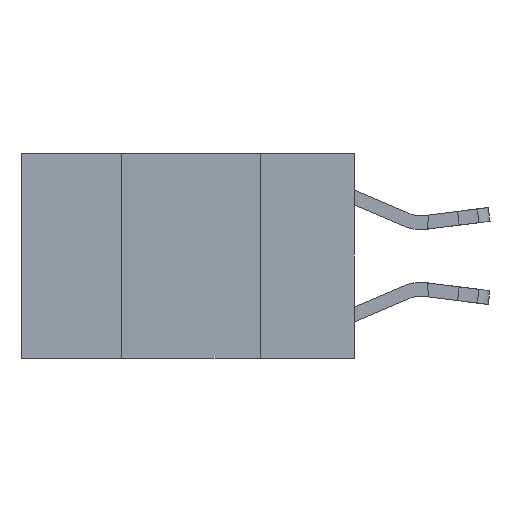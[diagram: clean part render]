
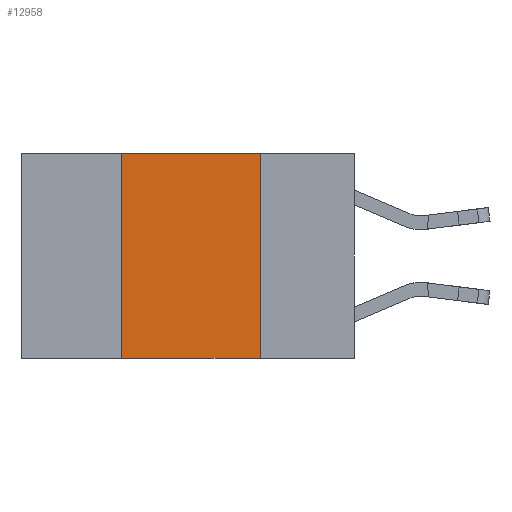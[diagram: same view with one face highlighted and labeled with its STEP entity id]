
A CAD part, left-side view. The second image highlights one B-rep face of the part: STEP entity #12958.
In plain terms, the highlighted planar face has unit normal (-1, 0, 0).
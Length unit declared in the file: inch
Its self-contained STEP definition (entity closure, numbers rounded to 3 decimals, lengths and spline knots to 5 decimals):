
#995 = CARTESIAN_POINT ( 'NONE',  ( 0., 0.42, 0. ) ) ;
#1064 = AXIS2_PLACEMENT_3D ( 'NONE', #13841, #3525, #10961 ) ;
#1070 = PLANE ( 'NONE',  #1064 ) ;
#2277 = ORIENTED_EDGE ( 'NONE', *, *, #11517, .F. ) ;
#2356 = FACE_OUTER_BOUND ( 'NONE', #9701, .T. ) ;
#2365 = ORIENTED_EDGE ( 'NONE', *, *, #9728, .T. ) ;
#2584 = ORIENTED_EDGE ( 'NONE', *, *, #3518, .F. ) ;
#2908 = DIRECTION ( 'NONE',  ( 0., 0., -1. ) ) ;
#2963 = CARTESIAN_POINT ( 'NONE',  ( 0., 0.42, 0. ) ) ;
#3089 = LINE ( 'NONE', #2963, #6203 ) ;
#3518 = EDGE_CURVE ( 'NONE', #4362, #11618, #12819, .T. ) ;
#3525 = DIRECTION ( 'NONE',  ( 1., 0., 0. ) ) ;
#4362 = VERTEX_POINT ( 'NONE', #995 ) ;
#4555 = LINE ( 'NONE', #10633, #12102 ) ;
#5373 = CARTESIAN_POINT ( 'NONE',  ( 0., 0.17, 0. ) ) ;
#5927 = CARTESIAN_POINT ( 'NONE',  ( 0., 0.42, -0.37 ) ) ;
#6156 = CARTESIAN_POINT ( 'NONE',  ( 0., 0.6, 0. ) ) ;
#6203 = VECTOR ( 'NONE', #10476, 39.37008 ) ;
#7369 = ORIENTED_EDGE ( 'NONE', *, *, #7930, .F. ) ;
#7440 = VERTEX_POINT ( 'NONE', #12605 ) ;
#7930 = EDGE_CURVE ( 'NONE', #11618, #7440, #10874, .T. ) ;
#9701 = EDGE_LOOP ( 'NONE', ( #7369, #2584, #2277, #2365 ) ) ;
#9728 = EDGE_CURVE ( 'NONE', #13743, #7440, #4555, .T. ) ;
#10385 = CARTESIAN_POINT ( 'NONE',  ( 0., 0.17, 0. ) ) ;
#10476 = DIRECTION ( 'NONE',  ( 0., 0., 1. ) ) ;
#10565 = VECTOR ( 'NONE', #2908, 39.37008 ) ;
#10633 = CARTESIAN_POINT ( 'NONE',  ( 0., 0.6, -0.37 ) ) ;
#10792 = DIRECTION ( 'NONE',  ( 0., -1., 0. ) ) ;
#10874 = LINE ( 'NONE', #10385, #10565 ) ;
#10961 = DIRECTION ( 'NONE',  ( 0., 0., -1. ) ) ;
#11517 = EDGE_CURVE ( 'NONE', #13743, #4362, #3089, .T. ) ;
#11570 = DIRECTION ( 'NONE',  ( 0., -1., 0. ) ) ;
#11618 = VERTEX_POINT ( 'NONE', #5373 ) ;
#12102 = VECTOR ( 'NONE', #11570, 39.37008 ) ;
#12503 = VECTOR ( 'NONE', #10792, 39.37008 ) ;
#12605 = CARTESIAN_POINT ( 'NONE',  ( 0., 0.17, -0.37 ) ) ;
#12819 = LINE ( 'NONE', #6156, #12503 ) ;
#12958 = ADVANCED_FACE ( 'NONE', ( #2356 ), #1070, .F. ) ;
#13743 = VERTEX_POINT ( 'NONE', #5927 ) ;
#13841 = CARTESIAN_POINT ( 'NONE',  ( 0., 0.6, 0. ) ) ;
